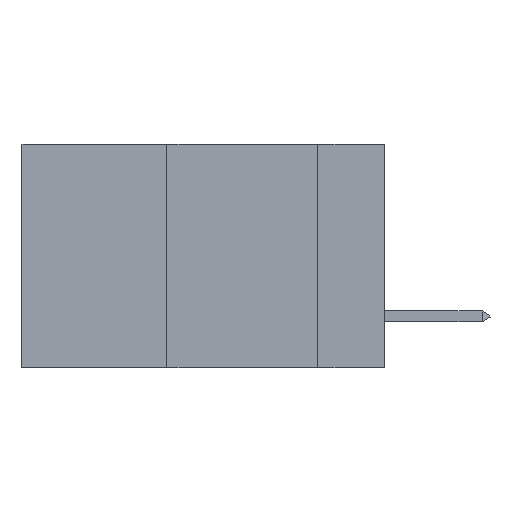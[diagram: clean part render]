
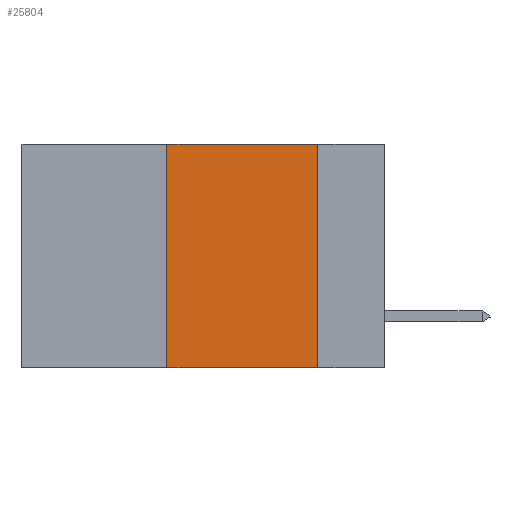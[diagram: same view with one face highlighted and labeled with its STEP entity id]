
A CAD part, left-side view. The second image highlights one B-rep face of the part: STEP entity #25804.
In plain terms, the highlighted planar face has unit normal (-1, 0, 0).
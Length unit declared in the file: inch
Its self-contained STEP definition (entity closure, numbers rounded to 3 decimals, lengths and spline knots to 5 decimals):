
#1767 = ORIENTED_EDGE ( 'NONE', *, *, #23962, .F. ) ;
#1971 = DIRECTION ( 'NONE',  ( 0., 0., 1. ) ) ;
#3738 = DIRECTION ( 'NONE',  ( 0., 0., -1. ) ) ;
#5556 = VECTOR ( 'NONE', #22805, 39.37008 ) ;
#5860 = ORIENTED_EDGE ( 'NONE', *, *, #23262, .F. ) ;
#6088 = AXIS2_PLACEMENT_3D ( 'NONE', #19519, #6650, #9351 ) ;
#6312 = CARTESIAN_POINT ( 'NONE',  ( 0., 0.36, -0.37 ) ) ;
#6650 = DIRECTION ( 'NONE',  ( 1., 0., 0. ) ) ;
#7176 = DIRECTION ( 'NONE',  ( 0., -1., 0. ) ) ;
#8984 = LINE ( 'NONE', #20403, #11463 ) ;
#9351 = DIRECTION ( 'NONE',  ( 0., 0., -1. ) ) ;
#11302 = VECTOR ( 'NONE', #3738, 39.37008 ) ;
#11463 = VECTOR ( 'NONE', #1971, 39.37008 ) ;
#11966 = ORIENTED_EDGE ( 'NONE', *, *, #14148, .T. ) ;
#13435 = CARTESIAN_POINT ( 'NONE',  ( 0., 0.36, 0. ) ) ;
#14148 = EDGE_CURVE ( 'NONE', #29337, #32610, #33330, .T. ) ;
#14523 = PLANE ( 'NONE',  #6088 ) ;
#15072 = EDGE_CURVE ( 'NONE', #24057, #32610, #18367, .T. ) ;
#15173 = CARTESIAN_POINT ( 'NONE',  ( 0., 0.6, -0.37 ) ) ;
#16719 = CARTESIAN_POINT ( 'NONE',  ( 0., 0.11, 0. ) ) ;
#18367 = LINE ( 'NONE', #16719, #11302 ) ;
#19519 = CARTESIAN_POINT ( 'NONE',  ( 0., 0.6, 0. ) ) ;
#20403 = CARTESIAN_POINT ( 'NONE',  ( 0., 0.36, 0. ) ) ;
#20989 = LINE ( 'NONE', #34107, #23053 ) ;
#22805 = DIRECTION ( 'NONE',  ( 0., -1., 0. ) ) ;
#23053 = VECTOR ( 'NONE', #7176, 39.37008 ) ;
#23262 = EDGE_CURVE ( 'NONE', #29337, #23534, #8984, .T. ) ;
#23534 = VERTEX_POINT ( 'NONE', #13435 ) ;
#23651 = ORIENTED_EDGE ( 'NONE', *, *, #15072, .F. ) ;
#23962 = EDGE_CURVE ( 'NONE', #23534, #24057, #20989, .T. ) ;
#24057 = VERTEX_POINT ( 'NONE', #31439 ) ;
#25804 = ADVANCED_FACE ( 'NONE', ( #33223 ), #14523, .F. ) ;
#28410 = EDGE_LOOP ( 'NONE', ( #23651, #1767, #5860, #11966 ) ) ;
#29337 = VERTEX_POINT ( 'NONE', #6312 ) ;
#31439 = CARTESIAN_POINT ( 'NONE',  ( 0., 0.11, 0. ) ) ;
#32610 = VERTEX_POINT ( 'NONE', #34217 ) ;
#33223 = FACE_OUTER_BOUND ( 'NONE', #28410, .T. ) ;
#33330 = LINE ( 'NONE', #15173, #5556 ) ;
#34107 = CARTESIAN_POINT ( 'NONE',  ( 0., 0.6, 0. ) ) ;
#34217 = CARTESIAN_POINT ( 'NONE',  ( 0., 0.11, -0.37 ) ) ;
